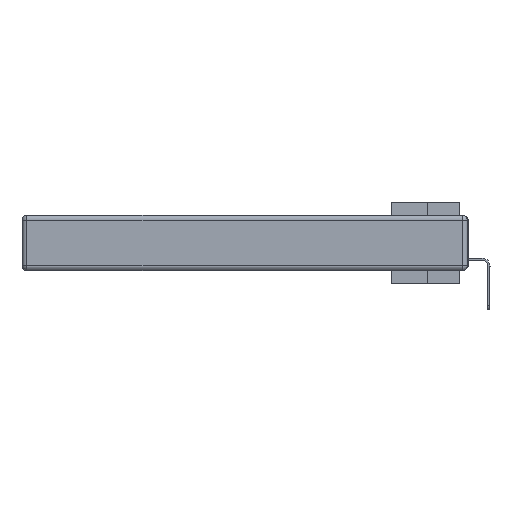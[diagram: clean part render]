
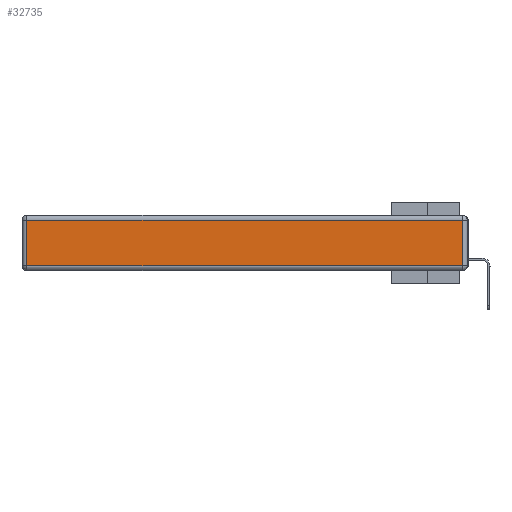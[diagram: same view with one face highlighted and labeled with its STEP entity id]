
A CAD part, left-side view. The second image highlights one B-rep face of the part: STEP entity #32735.
In plain terms, the highlighted planar face has unit normal (-1, 0, 0).
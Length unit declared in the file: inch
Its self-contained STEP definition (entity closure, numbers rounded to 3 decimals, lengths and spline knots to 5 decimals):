
#491 = ORIENTED_EDGE ( 'NONE', *, *, #21084, .T. ) ;
#2259 = VERTEX_POINT ( 'NONE', #4431 ) ;
#2387 = EDGE_LOOP ( 'NONE', ( #491, #37997, #26576, #25265 ) ) ;
#2726 = LINE ( 'NONE', #10254, #19890 ) ;
#4431 = CARTESIAN_POINT ( 'NONE',  ( 0., 2.72, -0.313 ) ) ;
#6158 = FACE_OUTER_BOUND ( 'NONE', #2387, .T. ) ;
#6165 = DIRECTION ( 'NONE',  ( 0., -1., 0. ) ) ;
#6792 = DIRECTION ( 'NONE',  ( 0., 0., -1. ) ) ;
#10254 = CARTESIAN_POINT ( 'NONE',  ( 0., 0.03, -0.343 ) ) ;
#13414 = VERTEX_POINT ( 'NONE', #34781 ) ;
#13670 = CARTESIAN_POINT ( 'NONE',  ( 0., 2.72, -0.03 ) ) ;
#13868 = LINE ( 'NONE', #33970, #31151 ) ;
#14173 = PLANE ( 'NONE',  #22646 ) ;
#15266 = CARTESIAN_POINT ( 'NONE',  ( 0., 0.03, -0.03 ) ) ;
#15481 = VERTEX_POINT ( 'NONE', #15266 ) ;
#15715 = LINE ( 'NONE', #22327, #28156 ) ;
#17922 = VECTOR ( 'NONE', #6792, 39.37008 ) ;
#19890 = VECTOR ( 'NONE', #28713, 39.37008 ) ;
#21084 = EDGE_CURVE ( 'NONE', #2259, #13414, #15715, .T. ) ;
#22327 = CARTESIAN_POINT ( 'NONE',  ( 0., 0., -0.313 ) ) ;
#22646 = AXIS2_PLACEMENT_3D ( 'NONE', #35550, #23394, #23658 ) ;
#23394 = DIRECTION ( 'NONE',  ( -1., 0., 0. ) ) ;
#23658 = DIRECTION ( 'NONE',  ( 0., 0., 1. ) ) ;
#25216 = VERTEX_POINT ( 'NONE', #13670 ) ;
#25265 = ORIENTED_EDGE ( 'NONE', *, *, #36270, .T. ) ;
#26576 = ORIENTED_EDGE ( 'NONE', *, *, #34365, .T. ) ;
#28156 = VECTOR ( 'NONE', #6165, 39.37008 ) ;
#28713 = DIRECTION ( 'NONE',  ( 0., 0., 1. ) ) ;
#29876 = DIRECTION ( 'NONE',  ( 0., 1., 0. ) ) ;
#30403 = EDGE_CURVE ( 'NONE', #13414, #15481, #2726, .T. ) ;
#31151 = VECTOR ( 'NONE', #29876, 39.37008 ) ;
#32735 = ADVANCED_FACE ( 'NONE', ( #6158 ), #14173, .T. ) ;
#33917 = CARTESIAN_POINT ( 'NONE',  ( 0., 2.72, -0.343 ) ) ;
#33970 = CARTESIAN_POINT ( 'NONE',  ( 0., 2.75, -0.03 ) ) ;
#34365 = EDGE_CURVE ( 'NONE', #15481, #25216, #13868, .T. ) ;
#34781 = CARTESIAN_POINT ( 'NONE',  ( 0., 0.03, -0.313 ) ) ;
#35550 = CARTESIAN_POINT ( 'NONE',  ( 0., 0., -0.343 ) ) ;
#36131 = LINE ( 'NONE', #33917, #17922 ) ;
#36270 = EDGE_CURVE ( 'NONE', #25216, #2259, #36131, .T. ) ;
#37997 = ORIENTED_EDGE ( 'NONE', *, *, #30403, .T. ) ;
